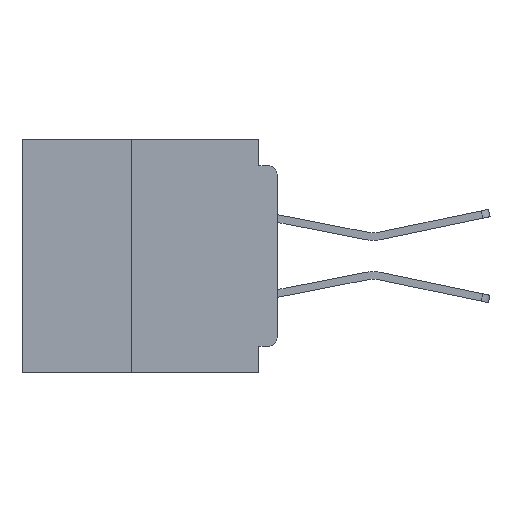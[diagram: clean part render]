
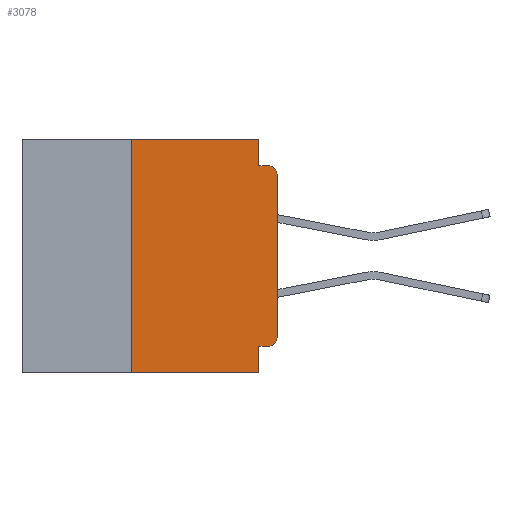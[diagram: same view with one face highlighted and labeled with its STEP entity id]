
A CAD part, left-side view. The second image highlights one B-rep face of the part: STEP entity #3078.
In plain terms, the highlighted planar face has unit normal (-1, 0, 0).
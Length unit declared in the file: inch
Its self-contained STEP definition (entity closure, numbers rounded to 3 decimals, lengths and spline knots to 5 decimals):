
#597 = CARTESIAN_POINT ( 'NONE',  ( 0., 0., 0. ) ) ;
#1672 = VERTEX_POINT ( 'NONE', #4170 ) ;
#1932 = AXIS2_PLACEMENT_3D ( 'NONE', #18306, #35167, #7765 ) ;
#2190 = ORIENTED_EDGE ( 'NONE', *, *, #29847, .T. ) ;
#2670 = VERTEX_POINT ( 'NONE', #24130 ) ;
#2823 = ORIENTED_EDGE ( 'NONE', *, *, #33628, .F. ) ;
#3078 = ADVANCED_FACE ( 'NONE', ( #24499 ), #16815, .F. ) ;
#3368 = CARTESIAN_POINT ( 'NONE',  ( 0., 0., -0.355 ) ) ;
#3774 = DIRECTION ( 'NONE',  ( 0., -1., 0. ) ) ;
#4170 = CARTESIAN_POINT ( 'NONE',  ( 0., 0., -0.34 ) ) ;
#4196 = LINE ( 'NONE', #35302, #11795 ) ;
#4351 = DIRECTION ( 'NONE',  ( -1., 0., 0. ) ) ;
#4367 = VECTOR ( 'NONE', #23432, 39.37008 ) ;
#4503 = CIRCLE ( 'NONE', #7307, 0.015 ) ;
#5749 = VECTOR ( 'NONE', #20568, 39.37008 ) ;
#6062 = AXIS2_PLACEMENT_3D ( 'NONE', #21423, #4351, #24305 ) ;
#6765 = CARTESIAN_POINT ( 'NONE',  ( 0., 0.25, -0.4 ) ) ;
#6981 = EDGE_LOOP ( 'NONE', ( #29882, #2190, #27699, #12968, #13919, #2823, #10450, #12181, #17987, #36304 ) ) ;
#7307 = AXIS2_PLACEMENT_3D ( 'NONE', #28421, #11354, #31278 ) ;
#7553 = LINE ( 'NONE', #11167, #13307 ) ;
#7721 = VERTEX_POINT ( 'NONE', #28483 ) ;
#7765 = DIRECTION ( 'NONE',  ( 0., 0., -1. ) ) ;
#8181 = DIRECTION ( 'NONE',  ( 0., 0., 1. ) ) ;
#10450 = ORIENTED_EDGE ( 'NONE', *, *, #33692, .T. ) ;
#11167 = CARTESIAN_POINT ( 'NONE',  ( 0., 0., -0.045 ) ) ;
#11354 = DIRECTION ( 'NONE',  ( -1., 0., 0. ) ) ;
#11795 = VECTOR ( 'NONE', #18188, 39.37008 ) ;
#12014 = VERTEX_POINT ( 'NONE', #21014 ) ;
#12181 = ORIENTED_EDGE ( 'NONE', *, *, #33908, .F. ) ;
#12968 = ORIENTED_EDGE ( 'NONE', *, *, #33577, .F. ) ;
#13307 = VECTOR ( 'NONE', #13990, 39.37008 ) ;
#13367 = CARTESIAN_POINT ( 'NONE',  ( 0., 0.031, 0. ) ) ;
#13919 = ORIENTED_EDGE ( 'NONE', *, *, #21998, .F. ) ;
#13990 = DIRECTION ( 'NONE',  ( 0., -1., 0. ) ) ;
#14126 = CARTESIAN_POINT ( 'NONE',  ( 0., 0.437, -0.4 ) ) ;
#15774 = VERTEX_POINT ( 'NONE', #6765 ) ;
#15976 = VERTEX_POINT ( 'NONE', #13367 ) ;
#16253 = CARTESIAN_POINT ( 'NONE',  ( 0., 0.031, 0. ) ) ;
#16815 = PLANE ( 'NONE',  #1932 ) ;
#16981 = DIRECTION ( 'NONE',  ( 0., -1., 0. ) ) ;
#17592 = VECTOR ( 'NONE', #8181, 39.37008 ) ;
#17987 = ORIENTED_EDGE ( 'NONE', *, *, #29674, .F. ) ;
#18178 = CARTESIAN_POINT ( 'NONE',  ( 0., 0.031, -0.355 ) ) ;
#18188 = DIRECTION ( 'NONE',  ( 0., 0., -1. ) ) ;
#18306 = CARTESIAN_POINT ( 'NONE',  ( 0., 0.437, 0. ) ) ;
#18466 = VECTOR ( 'NONE', #24880, 39.37008 ) ;
#18655 = VERTEX_POINT ( 'NONE', #35387 ) ;
#19926 = VECTOR ( 'NONE', #3774, 39.37008 ) ;
#20382 = LINE ( 'NONE', #3368, #4367 ) ;
#20568 = DIRECTION ( 'NONE',  ( 0., 0., 1. ) ) ;
#21014 = CARTESIAN_POINT ( 'NONE',  ( 0., 0.015, -0.355 ) ) ;
#21423 = CARTESIAN_POINT ( 'NONE',  ( 0., 0.015, -0.06 ) ) ;
#21614 = LINE ( 'NONE', #14126, #35891 ) ;
#21916 = CIRCLE ( 'NONE', #6062, 0.015 ) ;
#21998 = EDGE_CURVE ( 'NONE', #31139, #15976, #32500, .T. ) ;
#23402 = LINE ( 'NONE', #25258, #17592 ) ;
#23432 = DIRECTION ( 'NONE',  ( 0., 1., 0. ) ) ;
#24130 = CARTESIAN_POINT ( 'NONE',  ( 0., 0.015, -0.045 ) ) ;
#24305 = DIRECTION ( 'NONE',  ( 0., 0., -1. ) ) ;
#24499 = FACE_OUTER_BOUND ( 'NONE', #6981, .T. ) ;
#24880 = DIRECTION ( 'NONE',  ( 0., 0., -1. ) ) ;
#25258 = CARTESIAN_POINT ( 'NONE',  ( 0., 0.25, -0.4 ) ) ;
#27645 = LINE ( 'NONE', #597, #5749 ) ;
#27656 = CARTESIAN_POINT ( 'NONE',  ( 0., 0.25, 0. ) ) ;
#27699 = ORIENTED_EDGE ( 'NONE', *, *, #29498, .F. ) ;
#28421 = CARTESIAN_POINT ( 'NONE',  ( 0., 0.015, -0.34 ) ) ;
#28483 = CARTESIAN_POINT ( 'NONE',  ( 0., 0.031, -0.045 ) ) ;
#29072 = EDGE_CURVE ( 'NONE', #1672, #31636, #27645, .T. ) ;
#29452 = CARTESIAN_POINT ( 'NONE',  ( 0., 0.437, 0. ) ) ;
#29498 = EDGE_CURVE ( 'NONE', #7721, #2670, #7553, .T. ) ;
#29674 = EDGE_CURVE ( 'NONE', #12014, #32150, #20382, .T. ) ;
#29847 = EDGE_CURVE ( 'NONE', #31636, #2670, #21916, .T. ) ;
#29882 = ORIENTED_EDGE ( 'NONE', *, *, #29072, .T. ) ;
#30101 = CARTESIAN_POINT ( 'NONE',  ( 0., 0., -0.06 ) ) ;
#30121 = EDGE_CURVE ( 'NONE', #12014, #1672, #4503, .T. ) ;
#31139 = VERTEX_POINT ( 'NONE', #27656 ) ;
#31278 = DIRECTION ( 'NONE',  ( 0., 0., -1. ) ) ;
#31636 = VERTEX_POINT ( 'NONE', #30101 ) ;
#32150 = VERTEX_POINT ( 'NONE', #18178 ) ;
#32500 = LINE ( 'NONE', #29452, #19926 ) ;
#33577 = EDGE_CURVE ( 'NONE', #15976, #7721, #34586, .T. ) ;
#33628 = EDGE_CURVE ( 'NONE', #15774, #31139, #23402, .T. ) ;
#33692 = EDGE_CURVE ( 'NONE', #15774, #18655, #21614, .T. ) ;
#33908 = EDGE_CURVE ( 'NONE', #32150, #18655, #4196, .T. ) ;
#34586 = LINE ( 'NONE', #16253, #18466 ) ;
#35167 = DIRECTION ( 'NONE',  ( 1., 0., 0. ) ) ;
#35302 = CARTESIAN_POINT ( 'NONE',  ( 0., 0.031, -0.4 ) ) ;
#35387 = CARTESIAN_POINT ( 'NONE',  ( 0., 0.031, -0.4 ) ) ;
#35891 = VECTOR ( 'NONE', #16981, 39.37008 ) ;
#36304 = ORIENTED_EDGE ( 'NONE', *, *, #30121, .T. ) ;
